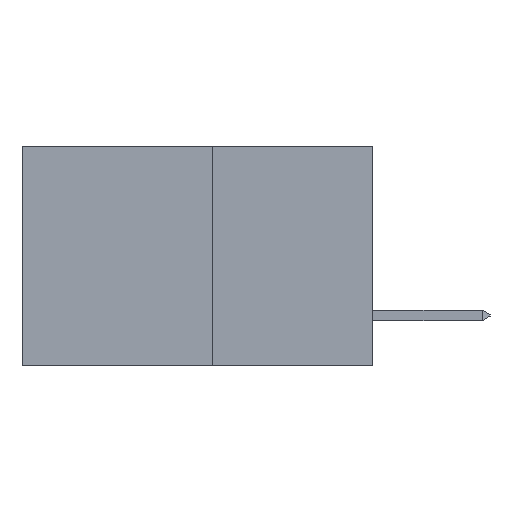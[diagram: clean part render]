
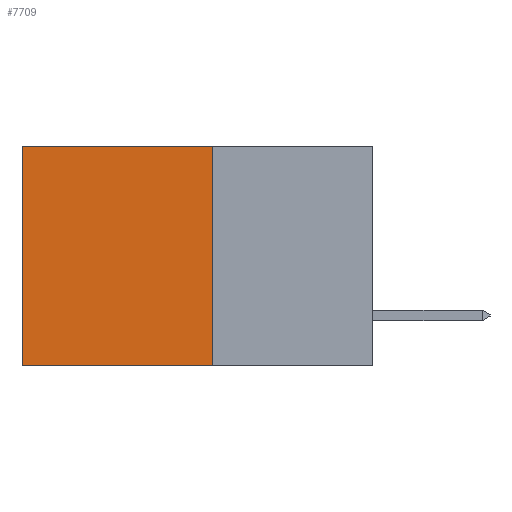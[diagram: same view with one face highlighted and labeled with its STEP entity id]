
A CAD part, left-side view. The second image highlights one B-rep face of the part: STEP entity #7709.
In plain terms, the highlighted planar face has unit normal (-1, 0, 0).
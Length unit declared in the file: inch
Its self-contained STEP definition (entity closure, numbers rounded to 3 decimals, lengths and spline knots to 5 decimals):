
#348 = ORIENTED_EDGE ( 'NONE', *, *, #8760, .T. ) ;
#1093 = CARTESIAN_POINT ( 'NONE',  ( 0.277, 0.59, 0. ) ) ;
#1477 = VERTEX_POINT ( 'NONE', #4642 ) ;
#1528 = DIRECTION ( 'NONE',  ( 0., 1., 0. ) ) ;
#1819 = CARTESIAN_POINT ( 'NONE',  ( 0.277, 0.27, 0. ) ) ;
#1917 = ORIENTED_EDGE ( 'NONE', *, *, #7874, .T. ) ;
#2812 = CARTESIAN_POINT ( 'NONE',  ( 0.277, 0.27, -0.37 ) ) ;
#3133 = ORIENTED_EDGE ( 'NONE', *, *, #9216, .F. ) ;
#3141 = PLANE ( 'NONE',  #11361 ) ;
#3279 = DIRECTION ( 'NONE',  ( 0., 0., -1. ) ) ;
#3302 = DIRECTION ( 'NONE',  ( 1., 0., 0. ) ) ;
#3408 = CARTESIAN_POINT ( 'NONE',  ( 0.277, 0.27, -0.37 ) ) ;
#3650 = VECTOR ( 'NONE', #11443, 39.37008 ) ;
#3690 = ORIENTED_EDGE ( 'NONE', *, *, #11839, .F. ) ;
#3959 = LINE ( 'NONE', #3408, #3650 ) ;
#4346 = LINE ( 'NONE', #5651, #6786 ) ;
#4642 = CARTESIAN_POINT ( 'NONE',  ( 0.277, 0.27, 0. ) ) ;
#4763 = EDGE_LOOP ( 'NONE', ( #1917, #3133, #3690, #348 ) ) ;
#4885 = LINE ( 'NONE', #11694, #9918 ) ;
#5004 = DIRECTION ( 'NONE',  ( 0., 1., 0. ) ) ;
#5651 = CARTESIAN_POINT ( 'NONE',  ( 0.277, 0.59, -0.37 ) ) ;
#5724 = DIRECTION ( 'NONE',  ( 0., 0., -1. ) ) ;
#6786 = VECTOR ( 'NONE', #5724, 39.37008 ) ;
#7709 = ADVANCED_FACE ( 'NONE', ( #8664 ), #3141, .F. ) ;
#7874 = EDGE_CURVE ( 'NONE', #8037, #11407, #4346, .T. ) ;
#8037 = VERTEX_POINT ( 'NONE', #1093 ) ;
#8244 = VECTOR ( 'NONE', #5004, 39.37008 ) ;
#8548 = LINE ( 'NONE', #1819, #8244 ) ;
#8664 = FACE_OUTER_BOUND ( 'NONE', #4763, .T. ) ;
#8760 = EDGE_CURVE ( 'NONE', #1477, #8037, #8548, .T. ) ;
#8794 = CARTESIAN_POINT ( 'NONE',  ( 0.277, 0.59, -0.37 ) ) ;
#9216 = EDGE_CURVE ( 'NONE', #10664, #11407, #4885, .T. ) ;
#9918 = VECTOR ( 'NONE', #1528, 39.37008 ) ;
#10664 = VERTEX_POINT ( 'NONE', #11061 ) ;
#11061 = CARTESIAN_POINT ( 'NONE',  ( 0.277, 0.27, -0.37 ) ) ;
#11361 = AXIS2_PLACEMENT_3D ( 'NONE', #2812, #3302, #3279 ) ;
#11407 = VERTEX_POINT ( 'NONE', #8794 ) ;
#11443 = DIRECTION ( 'NONE',  ( 0., 0., -1. ) ) ;
#11694 = CARTESIAN_POINT ( 'NONE',  ( 0.277, 0.27, -0.37 ) ) ;
#11839 = EDGE_CURVE ( 'NONE', #1477, #10664, #3959, .T. ) ;
